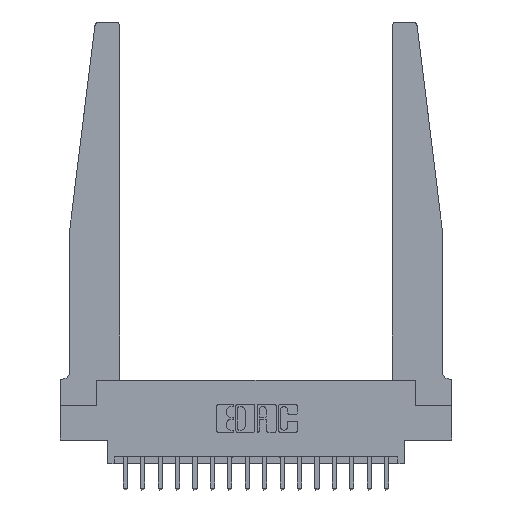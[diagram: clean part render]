
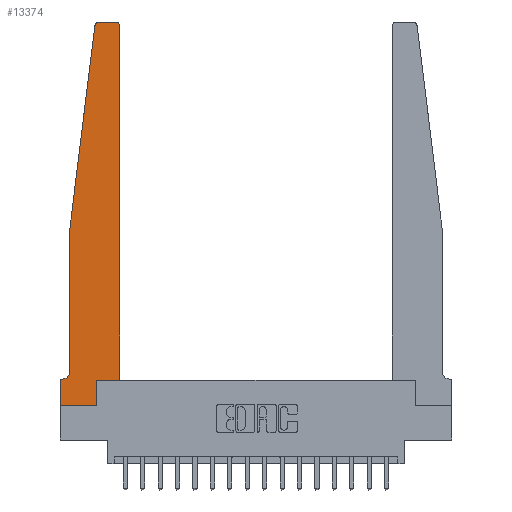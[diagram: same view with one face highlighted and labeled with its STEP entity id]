
A CAD part, top view. The second image highlights one B-rep face of the part: STEP entity #13374.
In plain terms, the highlighted planar face has unit normal (0, 0, 1).
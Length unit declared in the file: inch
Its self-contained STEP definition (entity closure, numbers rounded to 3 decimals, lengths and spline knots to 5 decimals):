
#370 = LINE ( 'NONE', #4089, #3398 ) ;
#542 = VERTEX_POINT ( 'NONE', #4860 ) ;
#732 = EDGE_CURVE ( 'NONE', #6471, #15258, #14234, .T. ) ;
#941 = VECTOR ( 'NONE', #959, 39.37008 ) ;
#959 = DIRECTION ( 'NONE',  ( -0.122, -0.992, 0. ) ) ;
#1567 = DIRECTION ( 'NONE',  ( 1., 0., 0. ) ) ;
#1573 = DIRECTION ( 'NONE',  ( 0., 0., 1. ) ) ;
#1596 = CARTESIAN_POINT ( 'NONE',  ( 0.395, 2.72, 0.37 ) ) ;
#1597 = ORIENTED_EDGE ( 'NONE', *, *, #6847, .T. ) ;
#1749 = CIRCLE ( 'NONE', #14039, 0.03 ) ;
#1851 = EDGE_CURVE ( 'NONE', #7356, #13039, #8455, .T. ) ;
#1868 = CARTESIAN_POINT ( 'NONE',  ( 0.425, 0.18, 0.37 ) ) ;
#2197 = CARTESIAN_POINT ( 'NONE',  ( 0., 0., 0.37 ) ) ;
#2369 = ORIENTED_EDGE ( 'NONE', *, *, #18475, .T. ) ;
#2787 = VERTEX_POINT ( 'NONE', #16607 ) ;
#2833 = FACE_OUTER_BOUND ( 'NONE', #7131, .T. ) ;
#2936 = DIRECTION ( 'NONE',  ( 0., 1., 0. ) ) ;
#2976 = LINE ( 'NONE', #13555, #14389 ) ;
#3139 = EDGE_CURVE ( 'NONE', #13100, #12498, #16585, .T. ) ;
#3357 = DIRECTION ( 'NONE',  ( 0., 0., 1. ) ) ;
#3398 = VECTOR ( 'NONE', #5620, 39.37008 ) ;
#3504 = VECTOR ( 'NONE', #5536, 39.37008 ) ;
#3721 = DIRECTION ( 'NONE',  ( 0., 0., -1. ) ) ;
#3777 = CARTESIAN_POINT ( 'NONE',  ( 0.24675, 2.72367, 0.37 ) ) ;
#4089 = CARTESIAN_POINT ( 'NONE',  ( 0.065, 0.1875, 0.37 ) ) ;
#4258 = EDGE_CURVE ( 'NONE', #18657, #11740, #15678, .T. ) ;
#4446 = VECTOR ( 'NONE', #6007, 39.37008 ) ;
#4504 = CARTESIAN_POINT ( 'NONE',  ( 0.2605, 0.18, 0.37 ) ) ;
#4677 = LINE ( 'NONE', #2197, #8655 ) ;
#4860 = CARTESIAN_POINT ( 'NONE',  ( 0.395, 2.75, 0.37 ) ) ;
#5068 = EDGE_CURVE ( 'NONE', #13039, #542, #1749, .T. ) ;
#5278 = DIRECTION ( 'NONE',  ( 0., -1., 0. ) ) ;
#5536 = DIRECTION ( 'NONE',  ( -1., 0., 0. ) ) ;
#5620 = DIRECTION ( 'NONE',  ( -1., 0., 0. ) ) ;
#6007 = DIRECTION ( 'NONE',  ( 0., 1., 0. ) ) ;
#6121 = CARTESIAN_POINT ( 'NONE',  ( 0.425, 0.18, 0.37 ) ) ;
#6146 = ORIENTED_EDGE ( 'NONE', *, *, #4258, .T. ) ;
#6367 = CARTESIAN_POINT ( 'NONE',  ( 0.425, 2.72, 0.37 ) ) ;
#6471 = VERTEX_POINT ( 'NONE', #13171 ) ;
#6847 = EDGE_CURVE ( 'NONE', #2787, #13100, #4677, .T. ) ;
#6962 = EDGE_CURVE ( 'NONE', #542, #6471, #7522, .T. ) ;
#7131 = EDGE_LOOP ( 'NONE', ( #14164, #10139, #16008, #6146, #9304, #2369, #1597, #11701, #16595, #14221, #11210, #14236 ) ) ;
#7356 = VERTEX_POINT ( 'NONE', #1868 ) ;
#7455 = CARTESIAN_POINT ( 'NONE',  ( 0.065, 1.25, 0.37 ) ) ;
#7522 = LINE ( 'NONE', #15803, #3504 ) ;
#7844 = PLANE ( 'NONE',  #8102 ) ;
#8102 = AXIS2_PLACEMENT_3D ( 'NONE', #12335, #3357, #13785 ) ;
#8246 = CARTESIAN_POINT ( 'NONE',  ( 0.015, 0.1875, 0.37 ) ) ;
#8455 = LINE ( 'NONE', #6121, #4446 ) ;
#8655 = VECTOR ( 'NONE', #5278, 39.37008 ) ;
#9056 = CARTESIAN_POINT ( 'NONE',  ( 0.2605, 0.18, 0.37 ) ) ;
#9115 = DIRECTION ( 'NONE',  ( 1., 0., 0. ) ) ;
#9304 = ORIENTED_EDGE ( 'NONE', *, *, #12564, .T. ) ;
#9486 = CARTESIAN_POINT ( 'NONE',  ( 0., 0., 0.37 ) ) ;
#9989 = CARTESIAN_POINT ( 'NONE',  ( 0.065, 1.25, 0.37 ) ) ;
#10139 = ORIENTED_EDGE ( 'NONE', *, *, #732, .T. ) ;
#10265 = AXIS2_PLACEMENT_3D ( 'NONE', #11118, #11215, #11172 ) ;
#10441 = DIRECTION ( 'NONE',  ( 0., -1., 0. ) ) ;
#10516 = VECTOR ( 'NONE', #10441, 39.37008 ) ;
#10560 = CARTESIAN_POINT ( 'NONE',  ( 0., 0., 0.37 ) ) ;
#10564 = CARTESIAN_POINT ( 'NONE',  ( 0.065, 1.25, 0.37 ) ) ;
#10586 = DIRECTION ( 'NONE',  ( 1., 0., 0. ) ) ;
#10984 = CARTESIAN_POINT ( 'NONE',  ( 0.065, 0.2375, 0.37 ) ) ;
#11118 = CARTESIAN_POINT ( 'NONE',  ( 0.27653, 2.72, 0.37 ) ) ;
#11172 = DIRECTION ( 'NONE',  ( 1., 0., 0. ) ) ;
#11210 = ORIENTED_EDGE ( 'NONE', *, *, #1851, .T. ) ;
#11215 = DIRECTION ( 'NONE',  ( 0., 0., 1. ) ) ;
#11225 = AXIS2_PLACEMENT_3D ( 'NONE', #12691, #3721, #14118 ) ;
#11520 = CIRCLE ( 'NONE', #11225, 0.05 ) ;
#11701 = ORIENTED_EDGE ( 'NONE', *, *, #3139, .T. ) ;
#11740 = VERTEX_POINT ( 'NONE', #10984 ) ;
#11859 = VERTEX_POINT ( 'NONE', #8246 ) ;
#11958 = EDGE_CURVE ( 'NONE', #15258, #18657, #12455, .T. ) ;
#12335 = CARTESIAN_POINT ( 'NONE',  ( 0., 0.1875, 0.37 ) ) ;
#12392 = VECTOR ( 'NONE', #10586, 39.37008 ) ;
#12455 = LINE ( 'NONE', #9989, #941 ) ;
#12498 = VERTEX_POINT ( 'NONE', #16742 ) ;
#12564 = EDGE_CURVE ( 'NONE', #11740, #11859, #11520, .T. ) ;
#12691 = CARTESIAN_POINT ( 'NONE',  ( 0.015, 0.2375, 0.37 ) ) ;
#13039 = VERTEX_POINT ( 'NONE', #6367 ) ;
#13100 = VERTEX_POINT ( 'NONE', #9486 ) ;
#13171 = CARTESIAN_POINT ( 'NONE',  ( 0.27653, 2.75, 0.37 ) ) ;
#13374 = ADVANCED_FACE ( 'NONE', ( #2833 ), #7844, .T. ) ;
#13555 = CARTESIAN_POINT ( 'NONE',  ( 0.425, 0.18, 0.37 ) ) ;
#13641 = EDGE_CURVE ( 'NONE', #12498, #14905, #18642, .T. ) ;
#13785 = DIRECTION ( 'NONE',  ( 1., 0., 0. ) ) ;
#14039 = AXIS2_PLACEMENT_3D ( 'NONE', #1596, #1573, #1567 ) ;
#14118 = DIRECTION ( 'NONE',  ( -1., 0., 0. ) ) ;
#14164 = ORIENTED_EDGE ( 'NONE', *, *, #6962, .T. ) ;
#14221 = ORIENTED_EDGE ( 'NONE', *, *, #16621, .T. ) ;
#14234 = CIRCLE ( 'NONE', #10265, 0.03 ) ;
#14236 = ORIENTED_EDGE ( 'NONE', *, *, #5068, .T. ) ;
#14389 = VECTOR ( 'NONE', #9115, 39.37008 ) ;
#14905 = VERTEX_POINT ( 'NONE', #9056 ) ;
#15258 = VERTEX_POINT ( 'NONE', #3777 ) ;
#15678 = LINE ( 'NONE', #10564, #10516 ) ;
#15803 = CARTESIAN_POINT ( 'NONE',  ( 0.25, 2.75, 0.37 ) ) ;
#16008 = ORIENTED_EDGE ( 'NONE', *, *, #11958, .T. ) ;
#16585 = LINE ( 'NONE', #10560, #12392 ) ;
#16595 = ORIENTED_EDGE ( 'NONE', *, *, #13641, .T. ) ;
#16607 = CARTESIAN_POINT ( 'NONE',  ( 0., 0.1875, 0.37 ) ) ;
#16621 = EDGE_CURVE ( 'NONE', #14905, #7356, #2976, .T. ) ;
#16742 = CARTESIAN_POINT ( 'NONE',  ( 0.2605, 0., 0.37 ) ) ;
#18219 = VECTOR ( 'NONE', #2936, 39.37008 ) ;
#18475 = EDGE_CURVE ( 'NONE', #11859, #2787, #370, .T. ) ;
#18642 = LINE ( 'NONE', #4504, #18219 ) ;
#18657 = VERTEX_POINT ( 'NONE', #7455 ) ;
